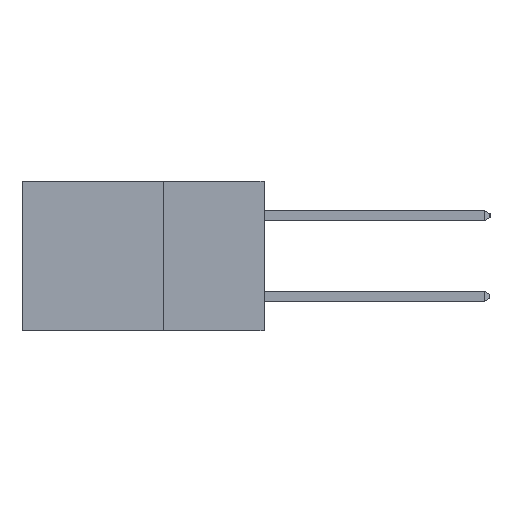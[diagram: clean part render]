
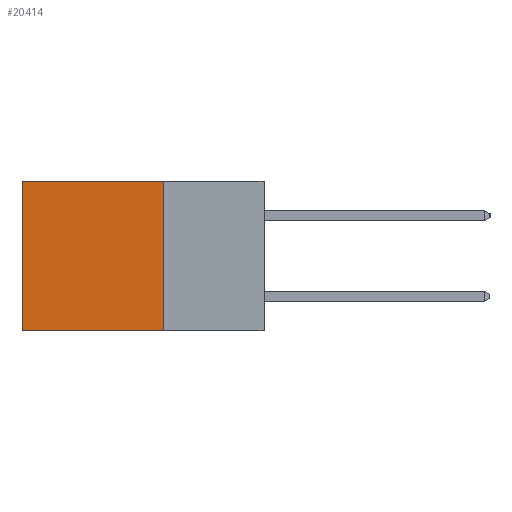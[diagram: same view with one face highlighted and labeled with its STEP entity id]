
A CAD part, left-side view. The second image highlights one B-rep face of the part: STEP entity #20414.
In plain terms, the highlighted planar face has unit normal (-1, 0, 0).
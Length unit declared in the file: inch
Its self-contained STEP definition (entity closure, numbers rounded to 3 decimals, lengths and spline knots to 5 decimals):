
#625 = LINE ( 'NONE', #7742, #14328 ) ;
#2391 = EDGE_CURVE ( 'NONE', #20165, #19624, #8852, .T. ) ;
#2698 = CARTESIAN_POINT ( 'NONE',  ( 0.2615, 0.6, -0.37 ) ) ;
#3976 = LINE ( 'NONE', #7057, #17537 ) ;
#4237 = DIRECTION ( 'NONE',  ( 1., 0., 0. ) ) ;
#4626 = ORIENTED_EDGE ( 'NONE', *, *, #21652, .T. ) ;
#5328 = LINE ( 'NONE', #2698, #22370 ) ;
#5815 = ORIENTED_EDGE ( 'NONE', *, *, #2391, .F. ) ;
#6157 = EDGE_CURVE ( 'NONE', #13297, #20165, #3976, .T. ) ;
#6703 = FACE_OUTER_BOUND ( 'NONE', #14039, .T. ) ;
#7015 = DIRECTION ( 'NONE',  ( 0., 0., -1. ) ) ;
#7057 = CARTESIAN_POINT ( 'NONE',  ( 0.2615, 0.25, -0.37 ) ) ;
#7742 = CARTESIAN_POINT ( 'NONE',  ( 0.2615, 0.25, 0. ) ) ;
#7785 = PLANE ( 'NONE',  #19585 ) ;
#7825 = VERTEX_POINT ( 'NONE', #18944 ) ;
#8852 = LINE ( 'NONE', #19545, #18190 ) ;
#9179 = CARTESIAN_POINT ( 'NONE',  ( 0.2615, 0.25, 0. ) ) ;
#9366 = CARTESIAN_POINT ( 'NONE',  ( 0.2615, 0.6, -0.37 ) ) ;
#10029 = ORIENTED_EDGE ( 'NONE', *, *, #18652, .T. ) ;
#10731 = ORIENTED_EDGE ( 'NONE', *, *, #6157, .F. ) ;
#13297 = VERTEX_POINT ( 'NONE', #9179 ) ;
#14039 = EDGE_LOOP ( 'NONE', ( #10029, #5815, #10731, #4626 ) ) ;
#14328 = VECTOR ( 'NONE', #16560, 39.37008 ) ;
#14674 = DIRECTION ( 'NONE',  ( 0., 1., 0. ) ) ;
#14854 = CARTESIAN_POINT ( 'NONE',  ( 0.2615, 0.25, -0.37 ) ) ;
#16560 = DIRECTION ( 'NONE',  ( 0., 1., 0. ) ) ;
#16606 = DIRECTION ( 'NONE',  ( 0., 0., -1. ) ) ;
#17537 = VECTOR ( 'NONE', #7015, 39.37008 ) ;
#18190 = VECTOR ( 'NONE', #14674, 39.37008 ) ;
#18652 = EDGE_CURVE ( 'NONE', #7825, #19624, #5328, .T. ) ;
#18681 = DIRECTION ( 'NONE',  ( 0., 0., -1. ) ) ;
#18944 = CARTESIAN_POINT ( 'NONE',  ( 0.2615, 0.6, 0. ) ) ;
#19545 = CARTESIAN_POINT ( 'NONE',  ( 0.2615, 0.25, -0.37 ) ) ;
#19585 = AXIS2_PLACEMENT_3D ( 'NONE', #14854, #4237, #16606 ) ;
#19624 = VERTEX_POINT ( 'NONE', #9366 ) ;
#20165 = VERTEX_POINT ( 'NONE', #22889 ) ;
#20414 = ADVANCED_FACE ( 'NONE', ( #6703 ), #7785, .F. ) ;
#21652 = EDGE_CURVE ( 'NONE', #13297, #7825, #625, .T. ) ;
#22370 = VECTOR ( 'NONE', #18681, 39.37008 ) ;
#22889 = CARTESIAN_POINT ( 'NONE',  ( 0.2615, 0.25, -0.37 ) ) ;
